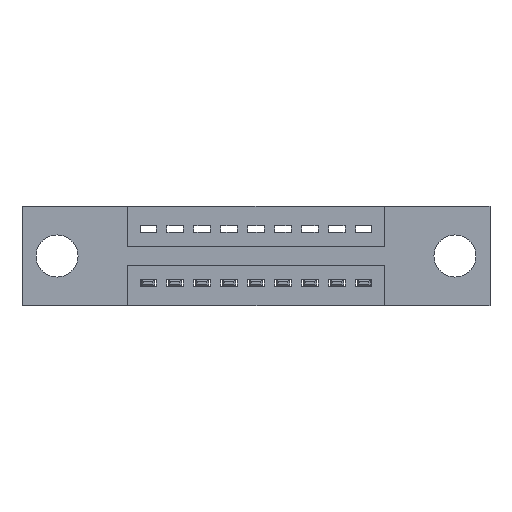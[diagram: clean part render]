
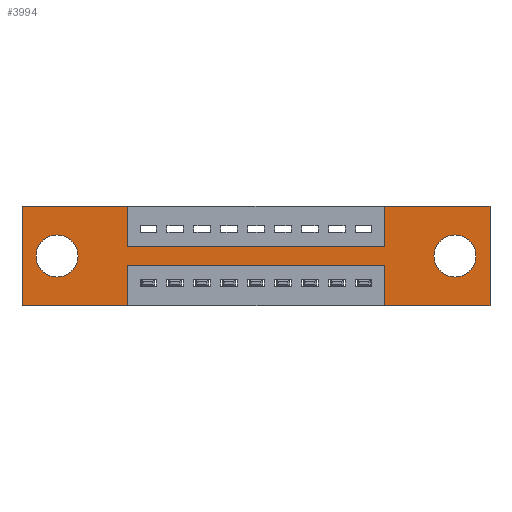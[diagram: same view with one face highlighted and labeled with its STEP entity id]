
A CAD part, front view. The second image highlights one B-rep face of the part: STEP entity #3994.
In plain terms, the highlighted planar face has unit normal (0, -1, 0).
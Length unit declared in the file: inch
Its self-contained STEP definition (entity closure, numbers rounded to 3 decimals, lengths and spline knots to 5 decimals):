
#28 = EDGE_CURVE ( 'NONE', #4514, #5389, #765, .T. ) ;
#44 = EDGE_CURVE ( 'NONE', #2479, #640, #6639, .T. ) ;
#120 = CIRCLE ( 'NONE', #2580, 0.078 ) ;
#122 = VECTOR ( 'NONE', #324, 39.37008 ) ;
#170 = VERTEX_POINT ( 'NONE', #5348 ) ;
#176 = FACE_BOUND ( 'NONE', #3203, .T. ) ;
#305 = VERTEX_POINT ( 'NONE', #9799 ) ;
#324 = DIRECTION ( 'NONE',  ( 0., 0., -1. ) ) ;
#391 = DIRECTION ( 'NONE',  ( 1., 0., 0. ) ) ;
#405 = ORIENTED_EDGE ( 'NONE', *, *, #6829, .F. ) ;
#549 = ORIENTED_EDGE ( 'NONE', *, *, #28, .F. ) ;
#629 = VECTOR ( 'NONE', #10557, 39.37008 ) ;
#640 = VERTEX_POINT ( 'NONE', #5095 ) ;
#758 = ORIENTED_EDGE ( 'NONE', *, *, #1203, .F. ) ;
#765 = LINE ( 'NONE', #7949, #122 ) ;
#890 = DIRECTION ( 'NONE',  ( 0., 1., 0. ) ) ;
#943 = VECTOR ( 'NONE', #6978, 39.37008 ) ;
#1020 = CARTESIAN_POINT ( 'NONE',  ( 0., 0., 0. ) ) ;
#1143 = EDGE_CURVE ( 'NONE', #3407, #8662, #1838, .T. ) ;
#1203 = EDGE_CURVE ( 'NONE', #11044, #2479, #6901, .T. ) ;
#1209 = FACE_BOUND ( 'NONE', #11030, .T. ) ;
#1675 = DIRECTION ( 'NONE',  ( 0., 0., 1. ) ) ;
#1833 = CARTESIAN_POINT ( 'NONE',  ( 0.3925, 0., -0.22 ) ) ;
#1838 = CIRCLE ( 'NONE', #4612, 0.078 ) ;
#1944 = VERTEX_POINT ( 'NONE', #7247 ) ;
#1960 = VECTOR ( 'NONE', #1675, 39.37008 ) ;
#1995 = ORIENTED_EDGE ( 'NONE', *, *, #9591, .F. ) ;
#2080 = DIRECTION ( 'NONE',  ( 0., 1., 0. ) ) ;
#2414 = CARTESIAN_POINT ( 'NONE',  ( 0., 0., 0. ) ) ;
#2479 = VERTEX_POINT ( 'NONE', #7722 ) ;
#2535 = CARTESIAN_POINT ( 'NONE',  ( 1.3425, 0., -0.37 ) ) ;
#2580 = AXIS2_PLACEMENT_3D ( 'NONE', #7600, #8420, #3312 ) ;
#2649 = VECTOR ( 'NONE', #9233, 39.37008 ) ;
#2678 = EDGE_CURVE ( 'NONE', #5389, #7903, #10453, .T. ) ;
#2722 = CARTESIAN_POINT ( 'NONE',  ( 0.13, 0., -0.263 ) ) ;
#2845 = CARTESIAN_POINT ( 'NONE',  ( 0., 0., -0.37 ) ) ;
#2893 = VERTEX_POINT ( 'NONE', #9059 ) ;
#2945 = DIRECTION ( 'NONE',  ( 0., 0., -1. ) ) ;
#3087 = VECTOR ( 'NONE', #4521, 39.37008 ) ;
#3160 = CARTESIAN_POINT ( 'NONE',  ( 0., 0., -0.37 ) ) ;
#3203 = EDGE_LOOP ( 'NONE', ( #4767, #8207 ) ) ;
#3312 = DIRECTION ( 'NONE',  ( 0., 0., 1. ) ) ;
#3407 = VERTEX_POINT ( 'NONE', #2722 ) ;
#3587 = LINE ( 'NONE', #2535, #2649 ) ;
#3644 = EDGE_CURVE ( 'NONE', #4370, #4514, #5489, .T. ) ;
#3838 = DIRECTION ( 'NONE',  ( -1., 0., 0. ) ) ;
#3980 = AXIS2_PLACEMENT_3D ( 'NONE', #3160, #10094, #6505 ) ;
#3994 = ADVANCED_FACE ( 'NONE', ( #176, #1209, #8971 ), #7363, .T. ) ;
#4106 = VECTOR ( 'NONE', #5975, 39.37008 ) ;
#4141 = CARTESIAN_POINT ( 'NONE',  ( 1.735, 0., 0. ) ) ;
#4370 = VERTEX_POINT ( 'NONE', #8915 ) ;
#4493 = VERTEX_POINT ( 'NONE', #10622 ) ;
#4514 = VERTEX_POINT ( 'NONE', #5488 ) ;
#4521 = DIRECTION ( 'NONE',  ( -1., 0., 0. ) ) ;
#4612 = AXIS2_PLACEMENT_3D ( 'NONE', #5268, #7863, #6929 ) ;
#4767 = ORIENTED_EDGE ( 'NONE', *, *, #9328, .T. ) ;
#4800 = LINE ( 'NONE', #8378, #10146 ) ;
#4934 = EDGE_CURVE ( 'NONE', #8645, #11044, #3587, .T. ) ;
#5000 = DIRECTION ( 'NONE',  ( 0., 0., -1. ) ) ;
#5095 = CARTESIAN_POINT ( 'NONE',  ( 0.3925, 0., -0.37 ) ) ;
#5114 = CARTESIAN_POINT ( 'NONE',  ( 0., 0., 0. ) ) ;
#5177 = LINE ( 'NONE', #10517, #629 ) ;
#5219 = VECTOR ( 'NONE', #8723, 39.37008 ) ;
#5268 = CARTESIAN_POINT ( 'NONE',  ( 0.13, 0., -0.185 ) ) ;
#5348 = CARTESIAN_POINT ( 'NONE',  ( 1.3425, 0., 0. ) ) ;
#5379 = ORIENTED_EDGE ( 'NONE', *, *, #44, .F. ) ;
#5380 = EDGE_CURVE ( 'NONE', #2893, #305, #8774, .T. ) ;
#5389 = VERTEX_POINT ( 'NONE', #5907 ) ;
#5488 = CARTESIAN_POINT ( 'NONE',  ( 0.3925, 0., 0. ) ) ;
#5489 = LINE ( 'NONE', #5114, #943 ) ;
#5512 = ORIENTED_EDGE ( 'NONE', *, *, #9882, .F. ) ;
#5862 = CARTESIAN_POINT ( 'NONE',  ( 0.13, 0., -0.107 ) ) ;
#5900 = VECTOR ( 'NONE', #391, 39.37008 ) ;
#5907 = CARTESIAN_POINT ( 'NONE',  ( 0.3925, 0., -0.15 ) ) ;
#5975 = DIRECTION ( 'NONE',  ( 0., 0., -1. ) ) ;
#6032 = ORIENTED_EDGE ( 'NONE', *, *, #8891, .F. ) ;
#6345 = ORIENTED_EDGE ( 'NONE', *, *, #4934, .F. ) ;
#6383 = EDGE_CURVE ( 'NONE', #8662, #3407, #120, .T. ) ;
#6498 = VECTOR ( 'NONE', #5000, 39.37008 ) ;
#6505 = DIRECTION ( 'NONE',  ( 0., 0., -1. ) ) ;
#6634 = DIRECTION ( 'NONE',  ( -1., 0., 0. ) ) ;
#6639 = LINE ( 'NONE', #10037, #6498 ) ;
#6824 = LINE ( 'NONE', #2845, #3087 ) ;
#6829 = EDGE_CURVE ( 'NONE', #7105, #4370, #9024, .T. ) ;
#6855 = CARTESIAN_POINT ( 'NONE',  ( 1.3425, 0., -0.37 ) ) ;
#6901 = LINE ( 'NONE', #1833, #8757 ) ;
#6929 = DIRECTION ( 'NONE',  ( 0., 0., 1. ) ) ;
#6978 = DIRECTION ( 'NONE',  ( 1., 0., 0. ) ) ;
#7003 = ORIENTED_EDGE ( 'NONE', *, *, #3644, .F. ) ;
#7105 = VERTEX_POINT ( 'NONE', #10789 ) ;
#7145 = ORIENTED_EDGE ( 'NONE', *, *, #5380, .F. ) ;
#7175 = CARTESIAN_POINT ( 'NONE',  ( 1.605, 0., -0.185 ) ) ;
#7247 = CARTESIAN_POINT ( 'NONE',  ( 1.605, 0., -0.263 ) ) ;
#7292 = ORIENTED_EDGE ( 'NONE', *, *, #1143, .T. ) ;
#7363 = PLANE ( 'NONE',  #3980 ) ;
#7495 = LINE ( 'NONE', #1020, #5219 ) ;
#7563 = CARTESIAN_POINT ( 'NONE',  ( 1.3425, 0., -0.15 ) ) ;
#7600 = CARTESIAN_POINT ( 'NONE',  ( 0.13, 0., -0.185 ) ) ;
#7722 = CARTESIAN_POINT ( 'NONE',  ( 0.3925, 0., -0.22 ) ) ;
#7863 = DIRECTION ( 'NONE',  ( 0., 1., 0. ) ) ;
#7903 = VERTEX_POINT ( 'NONE', #7563 ) ;
#7949 = CARTESIAN_POINT ( 'NONE',  ( 0.3925, 0., 0. ) ) ;
#8207 = ORIENTED_EDGE ( 'NONE', *, *, #10289, .T. ) ;
#8378 = CARTESIAN_POINT ( 'NONE',  ( 0., 0., -0.37 ) ) ;
#8420 = DIRECTION ( 'NONE',  ( 0., 1., 0. ) ) ;
#8440 = ORIENTED_EDGE ( 'NONE', *, *, #6383, .T. ) ;
#8467 = CARTESIAN_POINT ( 'NONE',  ( 1.605, 0., -0.185 ) ) ;
#8539 = CIRCLE ( 'NONE', #9520, 0.078 ) ;
#8645 = VERTEX_POINT ( 'NONE', #6855 ) ;
#8662 = VERTEX_POINT ( 'NONE', #5862 ) ;
#8717 = ORIENTED_EDGE ( 'NONE', *, *, #2678, .F. ) ;
#8723 = DIRECTION ( 'NONE',  ( 1., 0., 0. ) ) ;
#8757 = VECTOR ( 'NONE', #3838, 39.37008 ) ;
#8774 = LINE ( 'NONE', #4141, #4106 ) ;
#8834 = CIRCLE ( 'NONE', #9732, 0.078 ) ;
#8891 = EDGE_CURVE ( 'NONE', #170, #2893, #7495, .T. ) ;
#8915 = CARTESIAN_POINT ( 'NONE',  ( 0., 0., 0. ) ) ;
#8924 = EDGE_LOOP ( 'NONE', ( #5379, #758, #6345, #1995, #7145, #6032, #10495, #8717, #549, #7003, #405, #5512 ) ) ;
#8971 = FACE_OUTER_BOUND ( 'NONE', #8924, .T. ) ;
#9024 = LINE ( 'NONE', #2414, #1960 ) ;
#9059 = CARTESIAN_POINT ( 'NONE',  ( 1.735, 0., 0. ) ) ;
#9233 = DIRECTION ( 'NONE',  ( 0., 0., 1. ) ) ;
#9328 = EDGE_CURVE ( 'NONE', #4493, #1944, #8834, .T. ) ;
#9520 = AXIS2_PLACEMENT_3D ( 'NONE', #7175, #2080, #2945 ) ;
#9591 = EDGE_CURVE ( 'NONE', #305, #8645, #6824, .T. ) ;
#9732 = AXIS2_PLACEMENT_3D ( 'NONE', #8467, #890, #10981 ) ;
#9799 = CARTESIAN_POINT ( 'NONE',  ( 1.735, 0., -0.37 ) ) ;
#9841 = CARTESIAN_POINT ( 'NONE',  ( 0.3925, 0., -0.15 ) ) ;
#9882 = EDGE_CURVE ( 'NONE', #640, #7105, #4800, .T. ) ;
#10037 = CARTESIAN_POINT ( 'NONE',  ( 0.3925, 0., -0.37 ) ) ;
#10094 = DIRECTION ( 'NONE',  ( 0., -1., 0. ) ) ;
#10099 = CARTESIAN_POINT ( 'NONE',  ( 1.3425, 0., -0.22 ) ) ;
#10146 = VECTOR ( 'NONE', #6634, 39.37008 ) ;
#10289 = EDGE_CURVE ( 'NONE', #1944, #4493, #8539, .T. ) ;
#10453 = LINE ( 'NONE', #9841, #5900 ) ;
#10495 = ORIENTED_EDGE ( 'NONE', *, *, #10825, .F. ) ;
#10517 = CARTESIAN_POINT ( 'NONE',  ( 1.3425, 0., 0. ) ) ;
#10557 = DIRECTION ( 'NONE',  ( 0., 0., 1. ) ) ;
#10622 = CARTESIAN_POINT ( 'NONE',  ( 1.605, 0., -0.107 ) ) ;
#10789 = CARTESIAN_POINT ( 'NONE',  ( 0., 0., -0.37 ) ) ;
#10825 = EDGE_CURVE ( 'NONE', #7903, #170, #5177, .T. ) ;
#10981 = DIRECTION ( 'NONE',  ( 0., 0., -1. ) ) ;
#11030 = EDGE_LOOP ( 'NONE', ( #8440, #7292 ) ) ;
#11044 = VERTEX_POINT ( 'NONE', #10099 ) ;
